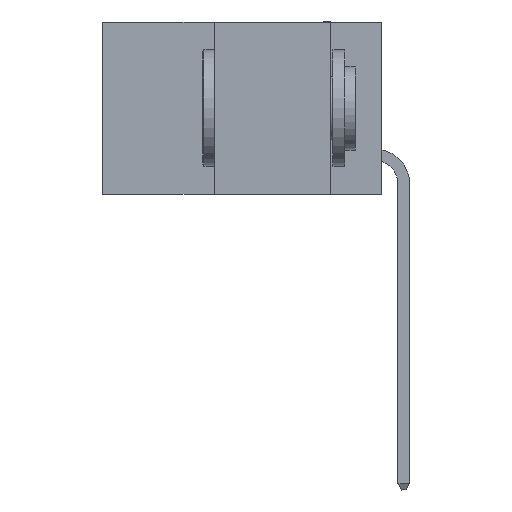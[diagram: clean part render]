
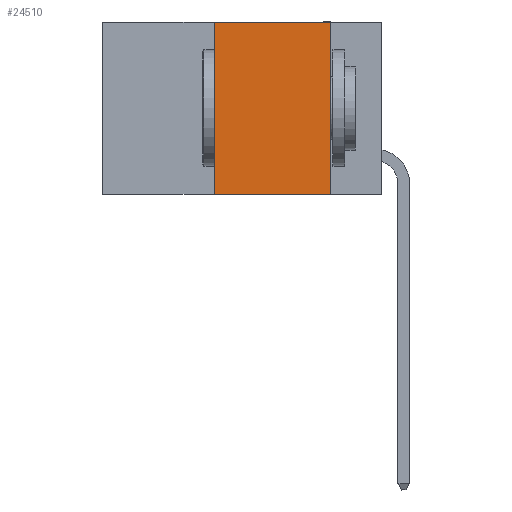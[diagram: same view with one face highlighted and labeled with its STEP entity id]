
A CAD part, left-side view. The second image highlights one B-rep face of the part: STEP entity #24510.
In plain terms, the highlighted planar face has unit normal (-1, 0, 0).
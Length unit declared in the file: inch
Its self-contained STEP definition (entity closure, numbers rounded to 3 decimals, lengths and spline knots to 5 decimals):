
#776 = VERTEX_POINT ( 'NONE', #27924 ) ;
#3982 = CARTESIAN_POINT ( 'NONE',  ( 0., 0.11, 0. ) ) ;
#4784 = DIRECTION ( 'NONE',  ( 0., -1., 0. ) ) ;
#5289 = ORIENTED_EDGE ( 'NONE', *, *, #17357, .T. ) ;
#6053 = LINE ( 'NONE', #3982, #23884 ) ;
#6367 = EDGE_LOOP ( 'NONE', ( #19283, #23622, #38501, #5289 ) ) ;
#6686 = CARTESIAN_POINT ( 'NONE',  ( 0., 0.36, 0. ) ) ;
#7666 = CARTESIAN_POINT ( 'NONE',  ( 0., 0.6, 0. ) ) ;
#8634 = VECTOR ( 'NONE', #4784, 39.37008 ) ;
#10647 = DIRECTION ( 'NONE',  ( 0., -1., 0. ) ) ;
#10860 = CARTESIAN_POINT ( 'NONE',  ( 0., 0.6, -0.37 ) ) ;
#11993 = VERTEX_POINT ( 'NONE', #36302 ) ;
#15354 = LINE ( 'NONE', #10860, #8634 ) ;
#15497 = DIRECTION ( 'NONE',  ( 0., 0., 1. ) ) ;
#15532 = VERTEX_POINT ( 'NONE', #6686 ) ;
#15567 = AXIS2_PLACEMENT_3D ( 'NONE', #36663, #24672, #18480 ) ;
#16320 = CARTESIAN_POINT ( 'NONE',  ( 0., 0.36, -0.37 ) ) ;
#17171 = EDGE_CURVE ( 'NONE', #15532, #776, #34587, .T. ) ;
#17357 = EDGE_CURVE ( 'NONE', #34577, #11993, #15354, .T. ) ;
#18480 = DIRECTION ( 'NONE',  ( 0., 0., -1. ) ) ;
#19283 = ORIENTED_EDGE ( 'NONE', *, *, #19996, .F. ) ;
#19996 = EDGE_CURVE ( 'NONE', #776, #11993, #6053, .T. ) ;
#21621 = VECTOR ( 'NONE', #15497, 39.37008 ) ;
#22039 = DIRECTION ( 'NONE',  ( 0., 0., -1. ) ) ;
#23622 = ORIENTED_EDGE ( 'NONE', *, *, #17171, .F. ) ;
#23884 = VECTOR ( 'NONE', #22039, 39.37008 ) ;
#24510 = ADVANCED_FACE ( 'NONE', ( #30151 ), #33837, .F. ) ;
#24672 = DIRECTION ( 'NONE',  ( 1., 0., 0. ) ) ;
#26428 = LINE ( 'NONE', #28021, #21621 ) ;
#26867 = VECTOR ( 'NONE', #10647, 39.37008 ) ;
#27924 = CARTESIAN_POINT ( 'NONE',  ( 0., 0.11, 0. ) ) ;
#28021 = CARTESIAN_POINT ( 'NONE',  ( 0., 0.36, 0. ) ) ;
#30151 = FACE_OUTER_BOUND ( 'NONE', #6367, .T. ) ;
#30869 = EDGE_CURVE ( 'NONE', #34577, #15532, #26428, .T. ) ;
#33837 = PLANE ( 'NONE',  #15567 ) ;
#34577 = VERTEX_POINT ( 'NONE', #16320 ) ;
#34587 = LINE ( 'NONE', #7666, #26867 ) ;
#36302 = CARTESIAN_POINT ( 'NONE',  ( 0., 0.11, -0.37 ) ) ;
#36663 = CARTESIAN_POINT ( 'NONE',  ( 0., 0.6, 0. ) ) ;
#38501 = ORIENTED_EDGE ( 'NONE', *, *, #30869, .F. ) ;
